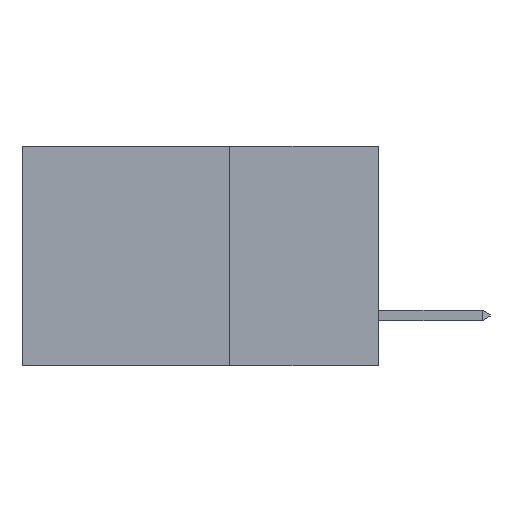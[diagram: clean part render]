
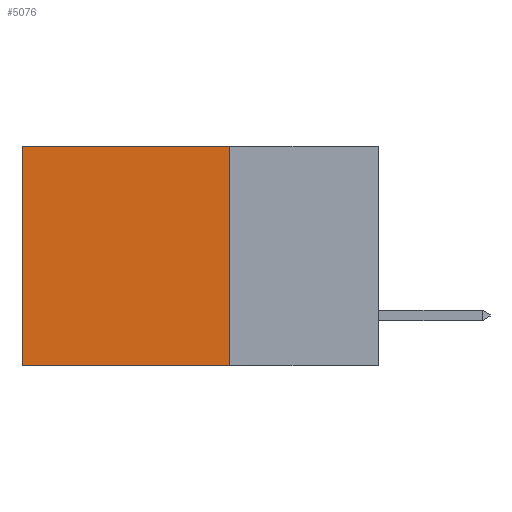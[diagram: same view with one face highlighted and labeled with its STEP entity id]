
A CAD part, left-side view. The second image highlights one B-rep face of the part: STEP entity #5076.
In plain terms, the highlighted planar face has unit normal (-1, 0, 0).
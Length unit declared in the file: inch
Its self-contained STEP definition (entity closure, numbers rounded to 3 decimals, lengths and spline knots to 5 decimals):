
#1313 = DIRECTION ( 'NONE',  ( 0., 1., 0. ) ) ;
#1454 = CARTESIAN_POINT ( 'NONE',  ( 0.2615, 0.6, -0.37 ) ) ;
#1571 = ORIENTED_EDGE ( 'NONE', *, *, #4715, .F. ) ;
#2446 = LINE ( 'NONE', #9477, #22306 ) ;
#4715 = EDGE_CURVE ( 'NONE', #12963, #12216, #20637, .T. ) ;
#5076 = ADVANCED_FACE ( 'NONE', ( #17936 ), #18830, .F. ) ;
#5078 = EDGE_CURVE ( 'NONE', #22006, #8817, #12859, .T. ) ;
#5086 = CARTESIAN_POINT ( 'NONE',  ( 0.2615, 0.25, -0.37 ) ) ;
#6161 = ORIENTED_EDGE ( 'NONE', *, *, #13585, .F. ) ;
#6445 = CARTESIAN_POINT ( 'NONE',  ( 0.2615, 0.25, -0.37 ) ) ;
#7979 = DIRECTION ( 'NONE',  ( 0., 0., -1. ) ) ;
#8817 = VERTEX_POINT ( 'NONE', #19691 ) ;
#9477 = CARTESIAN_POINT ( 'NONE',  ( 0.2615, 0.25, -0.37 ) ) ;
#10525 = VECTOR ( 'NONE', #22493, 39.37008 ) ;
#11072 = EDGE_LOOP ( 'NONE', ( #23690, #1571, #6161, #11622 ) ) ;
#11622 = ORIENTED_EDGE ( 'NONE', *, *, #5078, .T. ) ;
#12216 = VERTEX_POINT ( 'NONE', #1454 ) ;
#12859 = LINE ( 'NONE', #18148, #24144 ) ;
#12963 = VERTEX_POINT ( 'NONE', #5086 ) ;
#13585 = EDGE_CURVE ( 'NONE', #22006, #12963, #2446, .T. ) ;
#14939 = LINE ( 'NONE', #24377, #10525 ) ;
#15561 = VECTOR ( 'NONE', #1313, 39.37008 ) ;
#16118 = CARTESIAN_POINT ( 'NONE',  ( 0.2615, 0.25, 0. ) ) ;
#16813 = EDGE_CURVE ( 'NONE', #8817, #12216, #14939, .T. ) ;
#17936 = FACE_OUTER_BOUND ( 'NONE', #11072, .T. ) ;
#18064 = DIRECTION ( 'NONE',  ( 0., 1., 0. ) ) ;
#18148 = CARTESIAN_POINT ( 'NONE',  ( 0.2615, 0.25, 0. ) ) ;
#18384 = DIRECTION ( 'NONE',  ( 0., 0., -1. ) ) ;
#18510 = DIRECTION ( 'NONE',  ( 1., 0., 0. ) ) ;
#18632 = CARTESIAN_POINT ( 'NONE',  ( 0.2615, 0.25, -0.37 ) ) ;
#18830 = PLANE ( 'NONE',  #22512 ) ;
#19691 = CARTESIAN_POINT ( 'NONE',  ( 0.2615, 0.6, 0. ) ) ;
#20637 = LINE ( 'NONE', #6445, #15561 ) ;
#22006 = VERTEX_POINT ( 'NONE', #16118 ) ;
#22306 = VECTOR ( 'NONE', #7979, 39.37008 ) ;
#22493 = DIRECTION ( 'NONE',  ( 0., 0., -1. ) ) ;
#22512 = AXIS2_PLACEMENT_3D ( 'NONE', #18632, #18510, #18384 ) ;
#23690 = ORIENTED_EDGE ( 'NONE', *, *, #16813, .T. ) ;
#24144 = VECTOR ( 'NONE', #18064, 39.37008 ) ;
#24377 = CARTESIAN_POINT ( 'NONE',  ( 0.2615, 0.6, -0.37 ) ) ;
